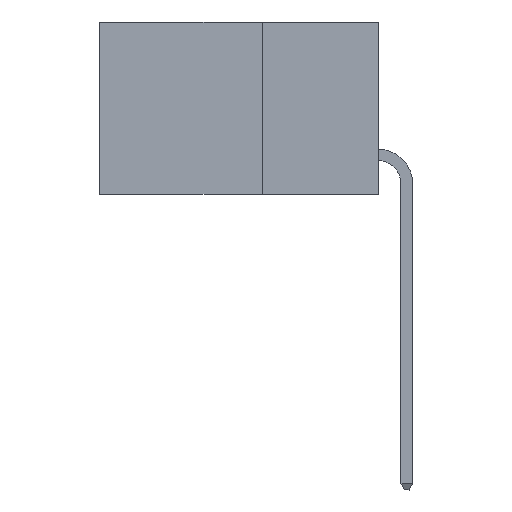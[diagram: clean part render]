
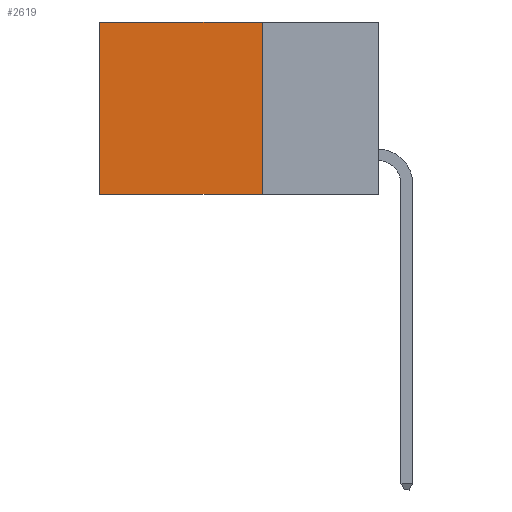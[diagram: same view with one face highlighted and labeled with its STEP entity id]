
A CAD part, left-side view. The second image highlights one B-rep face of the part: STEP entity #2619.
In plain terms, the highlighted planar face has unit normal (-1, 0, 0).
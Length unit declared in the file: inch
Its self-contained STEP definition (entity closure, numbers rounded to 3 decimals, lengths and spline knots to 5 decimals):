
#9 = ORIENTED_EDGE ( 'NONE', *, *, #656, .T. ) ;
#370 = LINE ( 'NONE', #11294, #5027 ) ;
#447 = CARTESIAN_POINT ( 'NONE',  ( 0.298, 0.25, 0. ) ) ;
#648 = CARTESIAN_POINT ( 'NONE',  ( 0.298, 0.6, 0. ) ) ;
#656 = EDGE_CURVE ( 'NONE', #8614, #1028, #2336, .T. ) ;
#836 = DIRECTION ( 'NONE',  ( 0., 0., -1. ) ) ;
#871 = CARTESIAN_POINT ( 'NONE',  ( 0.298, 0.25, 0. ) ) ;
#1028 = VERTEX_POINT ( 'NONE', #3403 ) ;
#1127 = VECTOR ( 'NONE', #6398, 39.37008 ) ;
#1743 = AXIS2_PLACEMENT_3D ( 'NONE', #871, #7839, #2887 ) ;
#2336 = LINE ( 'NONE', #10765, #5760 ) ;
#2619 = ADVANCED_FACE ( 'NONE', ( #4015 ), #3841, .F. ) ;
#2887 = DIRECTION ( 'NONE',  ( 0., 0., -1. ) ) ;
#3403 = CARTESIAN_POINT ( 'NONE',  ( 0.298, 0.6, -0.37 ) ) ;
#3448 = EDGE_CURVE ( 'NONE', #7610, #4712, #5824, .T. ) ;
#3841 = PLANE ( 'NONE',  #1743 ) ;
#4015 = FACE_OUTER_BOUND ( 'NONE', #8623, .T. ) ;
#4139 = CARTESIAN_POINT ( 'NONE',  ( 0.298, 0.25, 0. ) ) ;
#4267 = CARTESIAN_POINT ( 'NONE',  ( 0.298, 0.25, -0.37 ) ) ;
#4712 = VERTEX_POINT ( 'NONE', #4267 ) ;
#5027 = VECTOR ( 'NONE', #7420, 39.37008 ) ;
#5347 = VECTOR ( 'NONE', #9937, 39.37008 ) ;
#5760 = VECTOR ( 'NONE', #836, 39.37008 ) ;
#5824 = LINE ( 'NONE', #4139, #5347 ) ;
#6121 = LINE ( 'NONE', #447, #1127 ) ;
#6398 = DIRECTION ( 'NONE',  ( 0., 1., 0. ) ) ;
#7420 = DIRECTION ( 'NONE',  ( 0., 1., 0. ) ) ;
#7610 = VERTEX_POINT ( 'NONE', #10245 ) ;
#7839 = DIRECTION ( 'NONE',  ( 1., 0., 0. ) ) ;
#8614 = VERTEX_POINT ( 'NONE', #648 ) ;
#8623 = EDGE_LOOP ( 'NONE', ( #9, #9587, #10467, #10034 ) ) ;
#9536 = EDGE_CURVE ( 'NONE', #7610, #8614, #6121, .T. ) ;
#9539 = EDGE_CURVE ( 'NONE', #4712, #1028, #370, .T. ) ;
#9587 = ORIENTED_EDGE ( 'NONE', *, *, #9539, .F. ) ;
#9937 = DIRECTION ( 'NONE',  ( 0., 0., -1. ) ) ;
#10034 = ORIENTED_EDGE ( 'NONE', *, *, #9536, .T. ) ;
#10245 = CARTESIAN_POINT ( 'NONE',  ( 0.298, 0.25, 0. ) ) ;
#10467 = ORIENTED_EDGE ( 'NONE', *, *, #3448, .F. ) ;
#10765 = CARTESIAN_POINT ( 'NONE',  ( 0.298, 0.6, 0. ) ) ;
#11294 = CARTESIAN_POINT ( 'NONE',  ( 0.298, 0.25, -0.37 ) ) ;
